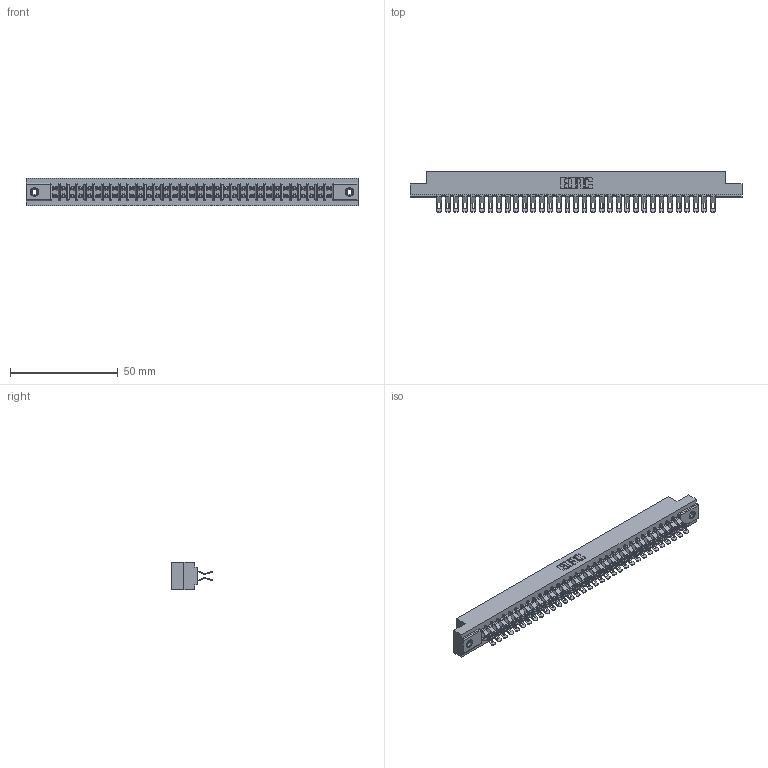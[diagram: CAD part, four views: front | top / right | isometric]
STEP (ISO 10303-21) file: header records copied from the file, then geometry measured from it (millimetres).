
FILE_DESCRIPTION (( 'STEP AP203' ), '1' );
FILE_NAME ('307-066-555-208.STEP', '2019-09-06T18:16:57', ( '' ), ( '' ), 'SwSTEP 2.0', 'SolidWorks 2016', '' );
FILE_SCHEMA (( 'CONFIG_CONTROL_DESIGN' ));
Length unit declared in the file: inch
Products named in the file (4): 307-066-555-208; 307 Part_.156 Dia Mounting Holes; 307-290-001_555; 345-250-001_345-250-003-102
Assembly tree (69 placements, depth 2):
  307-066-555-208
    307 Part_.156 Dia Mounting Holes
    307-290-001_555  x66
    345-250-001_345-250-003-102  x2
Bounding box: 153.77 x 18.75 x 12.7 mm (x, y, z)
Volume: 16478.1 mm3; surface area: 21092.3 mm2
Topology: 69 solids, 69 shells, 4238 faces, 12405 edges, 8082 vertices
Faces by surface type: plane 2346, cylinder 1808, sphere 68, cone 12, torus 4
Entity records: 32178 total; most frequent: CARTESIAN_POINT 5256, ORIENTED_EDGE 5204, DIRECTION 5168, EDGE_CURVE 2602, LINE 1980, VECTOR 1980, VERTEX_POINT 1682, AXIS2_PLACEMENT_3D 1594
